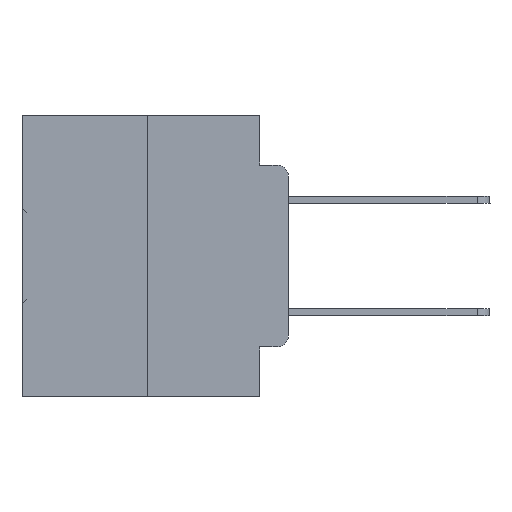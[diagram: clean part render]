
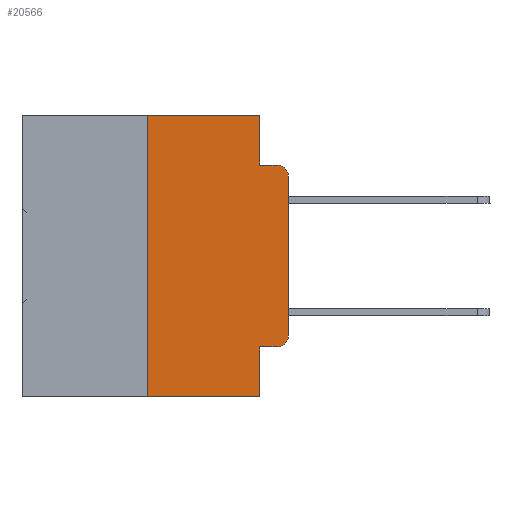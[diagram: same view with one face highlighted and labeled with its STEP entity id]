
A CAD part, left-side view. The second image highlights one B-rep face of the part: STEP entity #20566.
In plain terms, the highlighted planar face has unit normal (-1, 0, 0).
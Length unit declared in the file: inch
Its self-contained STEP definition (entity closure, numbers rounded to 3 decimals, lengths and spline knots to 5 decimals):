
#421 = CARTESIAN_POINT ( 'NONE',  ( 0., 0.02, -0.1085 ) ) ;
#452 = CARTESIAN_POINT ( 'NONE',  ( 0., 0.25, 0. ) ) ;
#814 = DIRECTION ( 'NONE',  ( 0., -1., 0. ) ) ;
#879 = VECTOR ( 'NONE', #15881, 39.37008 ) ;
#983 = LINE ( 'NONE', #452, #27855 ) ;
#1147 = ORIENTED_EDGE ( 'NONE', *, *, #1459, .F. ) ;
#1355 = ORIENTED_EDGE ( 'NONE', *, *, #11960, .T. ) ;
#1459 = EDGE_CURVE ( 'NONE', #4665, #28396, #10623, .T. ) ;
#1705 = DIRECTION ( 'NONE',  ( 0., 0., -1. ) ) ;
#2200 = LINE ( 'NONE', #24227, #26812 ) ;
#3334 = PLANE ( 'NONE',  #22870 ) ;
#3683 = FACE_OUTER_BOUND ( 'NONE', #15592, .T. ) ;
#3715 = VECTOR ( 'NONE', #25088, 39.37008 ) ;
#3825 = CARTESIAN_POINT ( 'NONE',  ( 0., 0.051, -0.4115 ) ) ;
#4007 = EDGE_CURVE ( 'NONE', #30654, #6037, #11098, .T. ) ;
#4456 = CARTESIAN_POINT ( 'NONE',  ( 0., 0.051, 0. ) ) ;
#4665 = VERTEX_POINT ( 'NONE', #17738 ) ;
#4744 = CARTESIAN_POINT ( 'NONE',  ( 0., 0.051, -0.0885 ) ) ;
#5974 = LINE ( 'NONE', #17521, #29667 ) ;
#6037 = VERTEX_POINT ( 'NONE', #34878 ) ;
#6217 = VERTEX_POINT ( 'NONE', #29725 ) ;
#6237 = EDGE_CURVE ( 'NONE', #6037, #34407, #2200, .T. ) ;
#6712 = VERTEX_POINT ( 'NONE', #27638 ) ;
#6816 = CARTESIAN_POINT ( 'NONE',  ( 0., 0.473, 0. ) ) ;
#7155 = CARTESIAN_POINT ( 'NONE',  ( 0., 0.02, -0.4115 ) ) ;
#7979 = ORIENTED_EDGE ( 'NONE', *, *, #12522, .T. ) ;
#8917 = CARTESIAN_POINT ( 'NONE',  ( 0., 0.02, -0.0885 ) ) ;
#9571 = DIRECTION ( 'NONE',  ( 0., 0., -1. ) ) ;
#10300 = DIRECTION ( 'NONE',  ( 0., 0., 1. ) ) ;
#10437 = LINE ( 'NONE', #33708, #3715 ) ;
#10553 = LINE ( 'NONE', #33463, #879 ) ;
#10623 = LINE ( 'NONE', #4744, #21875 ) ;
#10886 = DIRECTION ( 'NONE',  ( 0., 0., -1. ) ) ;
#10907 = CARTESIAN_POINT ( 'NONE',  ( 0., 0.051, 0. ) ) ;
#11063 = CARTESIAN_POINT ( 'NONE',  ( 0., 0.473, -0.5 ) ) ;
#11098 = CIRCLE ( 'NONE', #22778, 0.02 ) ;
#11431 = DIRECTION ( 'NONE',  ( 0., -1., 0. ) ) ;
#11960 = EDGE_CURVE ( 'NONE', #34548, #30654, #10553, .T. ) ;
#12522 = EDGE_CURVE ( 'NONE', #12914, #6217, #25351, .T. ) ;
#12914 = VERTEX_POINT ( 'NONE', #19022 ) ;
#13229 = VECTOR ( 'NONE', #11431, 39.37008 ) ;
#13474 = EDGE_CURVE ( 'NONE', #12914, #6712, #983, .T. ) ;
#13854 = CIRCLE ( 'NONE', #34325, 0.02 ) ;
#14025 = DIRECTION ( 'NONE',  ( 0., 0., -1. ) ) ;
#15468 = EDGE_CURVE ( 'NONE', #6712, #18529, #5974, .T. ) ;
#15592 = EDGE_LOOP ( 'NONE', ( #16269, #25259, #1147, #31785, #21387, #17736, #7979, #26312, #1355, #16108 ) ) ;
#15881 = DIRECTION ( 'NONE',  ( 0., -1., 0. ) ) ;
#16108 = ORIENTED_EDGE ( 'NONE', *, *, #4007, .T. ) ;
#16269 = ORIENTED_EDGE ( 'NONE', *, *, #6237, .T. ) ;
#16381 = LINE ( 'NONE', #4456, #27561 ) ;
#17521 = CARTESIAN_POINT ( 'NONE',  ( 0., 0.473, 0. ) ) ;
#17736 = ORIENTED_EDGE ( 'NONE', *, *, #13474, .F. ) ;
#17738 = CARTESIAN_POINT ( 'NONE',  ( 0., 0.051, -0.0885 ) ) ;
#18529 = VERTEX_POINT ( 'NONE', #10907 ) ;
#19022 = CARTESIAN_POINT ( 'NONE',  ( 0., 0.25, -0.5 ) ) ;
#20566 = ADVANCED_FACE ( 'NONE', ( #3683 ), #3334, .F. ) ;
#21387 = ORIENTED_EDGE ( 'NONE', *, *, #15468, .F. ) ;
#21608 = EDGE_CURVE ( 'NONE', #18529, #4665, #16381, .T. ) ;
#21875 = VECTOR ( 'NONE', #35210, 39.37008 ) ;
#22369 = CARTESIAN_POINT ( 'NONE',  ( 0., 0., -0.1085 ) ) ;
#22778 = AXIS2_PLACEMENT_3D ( 'NONE', #35455, #26639, #1705 ) ;
#22795 = DIRECTION ( 'NONE',  ( -1., 0., 0. ) ) ;
#22870 = AXIS2_PLACEMENT_3D ( 'NONE', #6816, #34677, #9571 ) ;
#24227 = CARTESIAN_POINT ( 'NONE',  ( 0., 0., 0. ) ) ;
#25088 = DIRECTION ( 'NONE',  ( 0., 0., -1. ) ) ;
#25259 = ORIENTED_EDGE ( 'NONE', *, *, #28873, .T. ) ;
#25351 = LINE ( 'NONE', #11063, #13229 ) ;
#25769 = DIRECTION ( 'NONE',  ( 0., 0., 1. ) ) ;
#26312 = ORIENTED_EDGE ( 'NONE', *, *, #34686, .F. ) ;
#26639 = DIRECTION ( 'NONE',  ( -1., 0., 0. ) ) ;
#26812 = VECTOR ( 'NONE', #10300, 39.37008 ) ;
#27561 = VECTOR ( 'NONE', #10886, 39.37008 ) ;
#27638 = CARTESIAN_POINT ( 'NONE',  ( 0., 0.25, 0. ) ) ;
#27855 = VECTOR ( 'NONE', #25769, 39.37008 ) ;
#28396 = VERTEX_POINT ( 'NONE', #8917 ) ;
#28873 = EDGE_CURVE ( 'NONE', #34407, #28396, #13854, .T. ) ;
#29667 = VECTOR ( 'NONE', #814, 39.37008 ) ;
#29725 = CARTESIAN_POINT ( 'NONE',  ( 0., 0.051, -0.5 ) ) ;
#30654 = VERTEX_POINT ( 'NONE', #7155 ) ;
#31785 = ORIENTED_EDGE ( 'NONE', *, *, #21608, .F. ) ;
#33463 = CARTESIAN_POINT ( 'NONE',  ( 0., 0.051, -0.4115 ) ) ;
#33708 = CARTESIAN_POINT ( 'NONE',  ( 0., 0.051, 0. ) ) ;
#34325 = AXIS2_PLACEMENT_3D ( 'NONE', #421, #22795, #14025 ) ;
#34407 = VERTEX_POINT ( 'NONE', #22369 ) ;
#34548 = VERTEX_POINT ( 'NONE', #3825 ) ;
#34677 = DIRECTION ( 'NONE',  ( 1., 0., 0. ) ) ;
#34686 = EDGE_CURVE ( 'NONE', #34548, #6217, #10437, .T. ) ;
#34878 = CARTESIAN_POINT ( 'NONE',  ( 0., 0., -0.3915 ) ) ;
#35210 = DIRECTION ( 'NONE',  ( 0., -1., 0. ) ) ;
#35455 = CARTESIAN_POINT ( 'NONE',  ( 0., 0.02, -0.3915 ) ) ;
